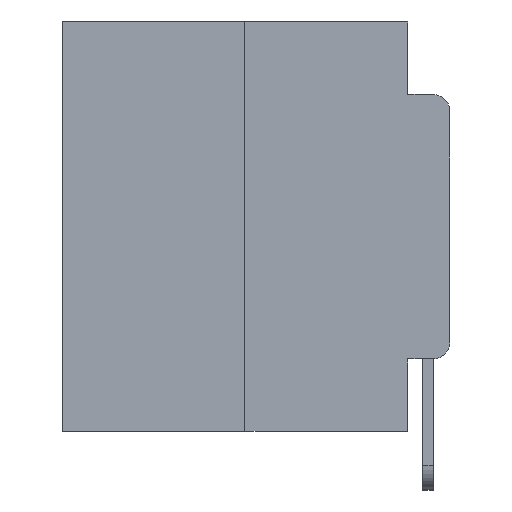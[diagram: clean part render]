
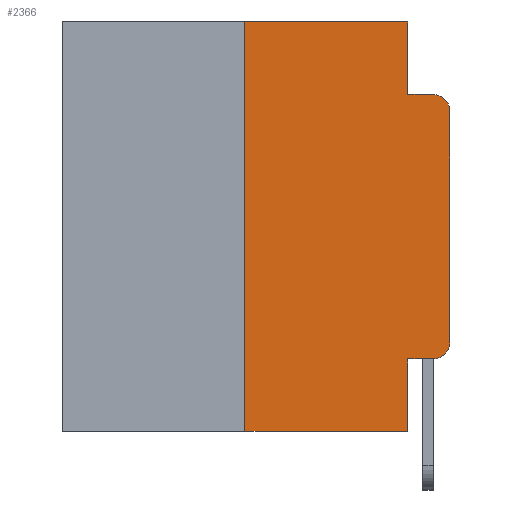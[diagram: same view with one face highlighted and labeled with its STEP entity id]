
A CAD part, left-side view. The second image highlights one B-rep face of the part: STEP entity #2366.
In plain terms, the highlighted planar face has unit normal (-1, 0, 0).
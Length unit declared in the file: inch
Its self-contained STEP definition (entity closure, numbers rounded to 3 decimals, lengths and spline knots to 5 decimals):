
#312 = LINE ( 'NONE', #8519, #21848 ) ;
#395 = EDGE_CURVE ( 'NONE', #20852, #17323, #7961, .T. ) ;
#429 = VERTEX_POINT ( 'NONE', #7158 ) ;
#607 = DIRECTION ( 'NONE',  ( 0., -1., 0. ) ) ;
#865 = VERTEX_POINT ( 'NONE', #25402 ) ;
#2262 = DIRECTION ( 'NONE',  ( 0., 0., -1. ) ) ;
#2340 = CARTESIAN_POINT ( 'NONE',  ( 0., 0., 0. ) ) ;
#2366 = ADVANCED_FACE ( 'NONE', ( #11170 ), #22436, .F. ) ;
#2873 = EDGE_CURVE ( 'NONE', #11637, #21021, #24303, .T. ) ;
#3490 = CIRCLE ( 'NONE', #5157, 0.02 ) ;
#3554 = CARTESIAN_POINT ( 'NONE',  ( 0., 0.051, 0. ) ) ;
#3600 = ORIENTED_EDGE ( 'NONE', *, *, #7681, .T. ) ;
#3693 = DIRECTION ( 'NONE',  ( 0., -1., 0. ) ) ;
#3826 = CARTESIAN_POINT ( 'NONE',  ( 0., 0.051, -0.4115 ) ) ;
#4042 = DIRECTION ( 'NONE',  ( 0., 0., -1. ) ) ;
#4233 = DIRECTION ( 'NONE',  ( 0., 0., 1. ) ) ;
#4364 = VERTEX_POINT ( 'NONE', #7364 ) ;
#4858 = ORIENTED_EDGE ( 'NONE', *, *, #6765, .T. ) ;
#5157 = AXIS2_PLACEMENT_3D ( 'NONE', #24736, #16259, #2262 ) ;
#5168 = CARTESIAN_POINT ( 'NONE',  ( 0., 0.473, 0. ) ) ;
#6064 = ORIENTED_EDGE ( 'NONE', *, *, #2873, .F. ) ;
#6433 = EDGE_LOOP ( 'NONE', ( #20044, #8658, #24656, #22742, #14592, #9542, #22078, #6064, #4858, #3600 ) ) ;
#6688 = LINE ( 'NONE', #18349, #21777 ) ;
#6765 = EDGE_CURVE ( 'NONE', #11637, #22695, #312, .T. ) ;
#6876 = VECTOR ( 'NONE', #607, 39.37008 ) ;
#7067 = DIRECTION ( 'NONE',  ( 0., -1., 0. ) ) ;
#7158 = CARTESIAN_POINT ( 'NONE',  ( 0., 0.25, -0.5 ) ) ;
#7364 = CARTESIAN_POINT ( 'NONE',  ( 0., 0.051, -0.0885 ) ) ;
#7368 = LINE ( 'NONE', #3554, #8344 ) ;
#7681 = EDGE_CURVE ( 'NONE', #22695, #865, #3490, .T. ) ;
#7704 = EDGE_CURVE ( 'NONE', #21596, #15685, #10907, .T. ) ;
#7961 = LINE ( 'NONE', #5168, #21100 ) ;
#8007 = EDGE_CURVE ( 'NONE', #429, #20852, #6688, .T. ) ;
#8307 = CARTESIAN_POINT ( 'NONE',  ( 0., 0.02, -0.1085 ) ) ;
#8344 = VECTOR ( 'NONE', #14039, 39.37008 ) ;
#8388 = DIRECTION ( 'NONE',  ( 0., 0., -1. ) ) ;
#8519 = CARTESIAN_POINT ( 'NONE',  ( 0., 0.051, -0.4115 ) ) ;
#8658 = ORIENTED_EDGE ( 'NONE', *, *, #7704, .T. ) ;
#9542 = ORIENTED_EDGE ( 'NONE', *, *, #8007, .F. ) ;
#9854 = CARTESIAN_POINT ( 'NONE',  ( 0., 0., -0.1085 ) ) ;
#10771 = LINE ( 'NONE', #19311, #6876 ) ;
#10824 = EDGE_CURVE ( 'NONE', #429, #21021, #15194, .T. ) ;
#10838 = VECTOR ( 'NONE', #20374, 39.37008 ) ;
#10907 = CIRCLE ( 'NONE', #11699, 0.02 ) ;
#11170 = FACE_OUTER_BOUND ( 'NONE', #6433, .T. ) ;
#11637 = VERTEX_POINT ( 'NONE', #3826 ) ;
#11699 = AXIS2_PLACEMENT_3D ( 'NONE', #8307, #16512, #8388 ) ;
#12333 = DIRECTION ( 'NONE',  ( 1., 0., 0. ) ) ;
#12797 = DIRECTION ( 'NONE',  ( 0., 0., 1. ) ) ;
#14039 = DIRECTION ( 'NONE',  ( 0., 0., -1. ) ) ;
#14113 = CARTESIAN_POINT ( 'NONE',  ( 0., 0.051, 0. ) ) ;
#14592 = ORIENTED_EDGE ( 'NONE', *, *, #395, .F. ) ;
#15194 = LINE ( 'NONE', #20017, #21325 ) ;
#15685 = VERTEX_POINT ( 'NONE', #25044 ) ;
#16259 = DIRECTION ( 'NONE',  ( -1., 0., 0. ) ) ;
#16325 = CARTESIAN_POINT ( 'NONE',  ( 0., 0.473, 0. ) ) ;
#16512 = DIRECTION ( 'NONE',  ( -1., 0., 0. ) ) ;
#17323 = VERTEX_POINT ( 'NONE', #14113 ) ;
#17568 = LINE ( 'NONE', #2340, #19507 ) ;
#18349 = CARTESIAN_POINT ( 'NONE',  ( 0., 0.25, 0. ) ) ;
#19165 = AXIS2_PLACEMENT_3D ( 'NONE', #16325, #12333, #4042 ) ;
#19311 = CARTESIAN_POINT ( 'NONE',  ( 0., 0.051, -0.0885 ) ) ;
#19507 = VECTOR ( 'NONE', #4233, 39.37008 ) ;
#20017 = CARTESIAN_POINT ( 'NONE',  ( 0., 0.473, -0.5 ) ) ;
#20044 = ORIENTED_EDGE ( 'NONE', *, *, #22402, .T. ) ;
#20374 = DIRECTION ( 'NONE',  ( 0., 0., -1. ) ) ;
#20852 = VERTEX_POINT ( 'NONE', #25873 ) ;
#21021 = VERTEX_POINT ( 'NONE', #21887 ) ;
#21100 = VECTOR ( 'NONE', #7067, 39.37008 ) ;
#21325 = VECTOR ( 'NONE', #3693, 39.37008 ) ;
#21593 = EDGE_CURVE ( 'NONE', #17323, #4364, #7368, .T. ) ;
#21596 = VERTEX_POINT ( 'NONE', #9854 ) ;
#21777 = VECTOR ( 'NONE', #12797, 39.37008 ) ;
#21848 = VECTOR ( 'NONE', #22867, 39.37008 ) ;
#21887 = CARTESIAN_POINT ( 'NONE',  ( 0., 0.051, -0.5 ) ) ;
#21890 = CARTESIAN_POINT ( 'NONE',  ( 0., 0.02, -0.4115 ) ) ;
#22078 = ORIENTED_EDGE ( 'NONE', *, *, #10824, .T. ) ;
#22402 = EDGE_CURVE ( 'NONE', #865, #21596, #17568, .T. ) ;
#22436 = PLANE ( 'NONE',  #19165 ) ;
#22695 = VERTEX_POINT ( 'NONE', #21890 ) ;
#22742 = ORIENTED_EDGE ( 'NONE', *, *, #21593, .F. ) ;
#22867 = DIRECTION ( 'NONE',  ( 0., -1., 0. ) ) ;
#24263 = EDGE_CURVE ( 'NONE', #4364, #15685, #10771, .T. ) ;
#24303 = LINE ( 'NONE', #24318, #10838 ) ;
#24318 = CARTESIAN_POINT ( 'NONE',  ( 0., 0.051, 0. ) ) ;
#24656 = ORIENTED_EDGE ( 'NONE', *, *, #24263, .F. ) ;
#24736 = CARTESIAN_POINT ( 'NONE',  ( 0., 0.02, -0.3915 ) ) ;
#25044 = CARTESIAN_POINT ( 'NONE',  ( 0., 0.02, -0.0885 ) ) ;
#25402 = CARTESIAN_POINT ( 'NONE',  ( 0., 0., -0.3915 ) ) ;
#25873 = CARTESIAN_POINT ( 'NONE',  ( 0., 0.25, 0. ) ) ;
